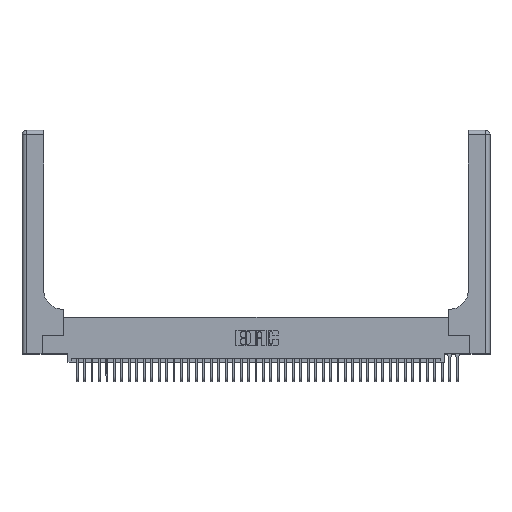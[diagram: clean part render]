
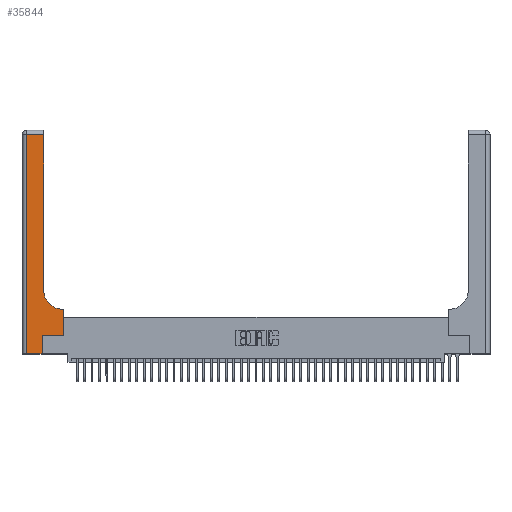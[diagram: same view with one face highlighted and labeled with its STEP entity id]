
A CAD part, top view. The second image highlights one B-rep face of the part: STEP entity #35844.
In plain terms, the highlighted planar face has unit normal (0, 0, 1).
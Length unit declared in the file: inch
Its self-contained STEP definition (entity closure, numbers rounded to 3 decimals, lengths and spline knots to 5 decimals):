
#328 = EDGE_CURVE ( 'NONE', #6774, #35759, #14251, .T. ) ;
#530 = CARTESIAN_POINT ( 'NONE',  ( 0.2915, 2.94, 0.37 ) ) ;
#949 = AXIS2_PLACEMENT_3D ( 'NONE', #9020, #31497, #12241 ) ;
#1760 = CARTESIAN_POINT ( 'NONE',  ( 0.2915, 3., 0.37 ) ) ;
#1807 = LINE ( 'NONE', #2555, #34940 ) ;
#2049 = VERTEX_POINT ( 'NONE', #25229 ) ;
#2165 = LINE ( 'NONE', #31288, #25928 ) ;
#2555 = CARTESIAN_POINT ( 'NONE',  ( 0., 2.94, 0.37 ) ) ;
#2743 = VERTEX_POINT ( 'NONE', #34445 ) ;
#3549 = EDGE_CURVE ( 'NONE', #31821, #21244, #12700, .T. ) ;
#4435 = EDGE_CURVE ( 'NONE', #2743, #31821, #18372, .T. ) ;
#5062 = CARTESIAN_POINT ( 'NONE',  ( 0.06, 0., 0.37 ) ) ;
#5066 = ORIENTED_EDGE ( 'NONE', *, *, #3549, .T. ) ;
#5427 = CARTESIAN_POINT ( 'NONE',  ( 0.2915, 0.85, 0.37 ) ) ;
#6137 = CARTESIAN_POINT ( 'NONE',  ( 0.269, 0.25, 0.37 ) ) ;
#6241 = DIRECTION ( 'NONE',  ( 0., 0., -1. ) ) ;
#6774 = VERTEX_POINT ( 'NONE', #39739 ) ;
#6879 = LINE ( 'NONE', #32406, #30571 ) ;
#7917 = EDGE_CURVE ( 'NONE', #20952, #32898, #6879, .T. ) ;
#9020 = CARTESIAN_POINT ( 'NONE',  ( 0.5415, 0.85, 0.37 ) ) ;
#9086 = CARTESIAN_POINT ( 'NONE',  ( 0.269, 0.25, 0.37 ) ) ;
#9711 = VECTOR ( 'NONE', #38661, 39.37008 ) ;
#10077 = DIRECTION ( 'NONE',  ( 1., 0., 0. ) ) ;
#10115 = EDGE_CURVE ( 'NONE', #19247, #20952, #1807, .T. ) ;
#10127 = DIRECTION ( 'NONE',  ( 0., -1., 0. ) ) ;
#10620 = LINE ( 'NONE', #1760, #27734 ) ;
#12241 = DIRECTION ( 'NONE',  ( 1., 0., 0. ) ) ;
#12306 = DIRECTION ( 'NONE',  ( -1., 0., 0. ) ) ;
#12700 = CIRCLE ( 'NONE', #949, 0.25 ) ;
#13233 = VECTOR ( 'NONE', #39094, 39.37008 ) ;
#13666 = EDGE_CURVE ( 'NONE', #35759, #2049, #20890, .T. ) ;
#14251 = LINE ( 'NONE', #23408, #13233 ) ;
#17146 = EDGE_LOOP ( 'NONE', ( #28143, #30082, #31790, #33692, #35648, #36331, #37935, #39816, #5066 ) ) ;
#17381 = CARTESIAN_POINT ( 'NONE',  ( 0.5415, 0.6, 0.37 ) ) ;
#18372 = LINE ( 'NONE', #32381, #9711 ) ;
#18657 = VECTOR ( 'NONE', #10077, 39.37008 ) ;
#19222 = FACE_OUTER_BOUND ( 'NONE', #17146, .T. ) ;
#19247 = VERTEX_POINT ( 'NONE', #530 ) ;
#20890 = LINE ( 'NONE', #6137, #35716 ) ;
#20952 = VERTEX_POINT ( 'NONE', #29818 ) ;
#21244 = VERTEX_POINT ( 'NONE', #5427 ) ;
#23408 = CARTESIAN_POINT ( 'NONE',  ( 0.269, 0., 0.37 ) ) ;
#24394 = DIRECTION ( 'NONE',  ( 0., 1., 0. ) ) ;
#25095 = AXIS2_PLACEMENT_3D ( 'NONE', #38088, #6241, #28776 ) ;
#25229 = CARTESIAN_POINT ( 'NONE',  ( 0.5585, 0.25, 0.37 ) ) ;
#25583 = PLANE ( 'NONE',  #25095 ) ;
#25928 = VECTOR ( 'NONE', #34418, 39.37008 ) ;
#26151 = CARTESIAN_POINT ( 'NONE',  ( 0., 0., 0.37 ) ) ;
#27734 = VECTOR ( 'NONE', #24394, 39.37008 ) ;
#28098 = LINE ( 'NONE', #26151, #18657 ) ;
#28143 = ORIENTED_EDGE ( 'NONE', *, *, #35033, .T. ) ;
#28776 = DIRECTION ( 'NONE',  ( -1., 0., 0. ) ) ;
#29818 = CARTESIAN_POINT ( 'NONE',  ( 0.06, 2.94, 0.37 ) ) ;
#30082 = ORIENTED_EDGE ( 'NONE', *, *, #10115, .T. ) ;
#30571 = VECTOR ( 'NONE', #10127, 39.37008 ) ;
#30614 = EDGE_CURVE ( 'NONE', #32898, #6774, #28098, .T. ) ;
#31288 = CARTESIAN_POINT ( 'NONE',  ( 0.5585, 0.25, 0.37 ) ) ;
#31497 = DIRECTION ( 'NONE',  ( 0., 0., -1. ) ) ;
#31790 = ORIENTED_EDGE ( 'NONE', *, *, #7917, .T. ) ;
#31821 = VERTEX_POINT ( 'NONE', #17381 ) ;
#31857 = DIRECTION ( 'NONE',  ( 1., 0., 0. ) ) ;
#32381 = CARTESIAN_POINT ( 'NONE',  ( 0.2915, 0.6, 0.37 ) ) ;
#32406 = CARTESIAN_POINT ( 'NONE',  ( 0.06, 3., 0.37 ) ) ;
#32898 = VERTEX_POINT ( 'NONE', #5062 ) ;
#33692 = ORIENTED_EDGE ( 'NONE', *, *, #30614, .T. ) ;
#34418 = DIRECTION ( 'NONE',  ( 0., 1., 0. ) ) ;
#34445 = CARTESIAN_POINT ( 'NONE',  ( 0.5585, 0.6, 0.37 ) ) ;
#34940 = VECTOR ( 'NONE', #12306, 39.37008 ) ;
#35033 = EDGE_CURVE ( 'NONE', #21244, #19247, #10620, .T. ) ;
#35648 = ORIENTED_EDGE ( 'NONE', *, *, #328, .T. ) ;
#35716 = VECTOR ( 'NONE', #31857, 39.37008 ) ;
#35759 = VERTEX_POINT ( 'NONE', #9086 ) ;
#35844 = ADVANCED_FACE ( 'NONE', ( #19222 ), #25583, .F. ) ;
#36331 = ORIENTED_EDGE ( 'NONE', *, *, #13666, .T. ) ;
#37935 = ORIENTED_EDGE ( 'NONE', *, *, #38422, .T. ) ;
#38088 = CARTESIAN_POINT ( 'NONE',  ( 0., 3., 0.37 ) ) ;
#38422 = EDGE_CURVE ( 'NONE', #2049, #2743, #2165, .T. ) ;
#38661 = DIRECTION ( 'NONE',  ( -1., 0., 0. ) ) ;
#39094 = DIRECTION ( 'NONE',  ( 0., 1., 0. ) ) ;
#39739 = CARTESIAN_POINT ( 'NONE',  ( 0.269, 0., 0.37 ) ) ;
#39816 = ORIENTED_EDGE ( 'NONE', *, *, #4435, .T. ) ;
